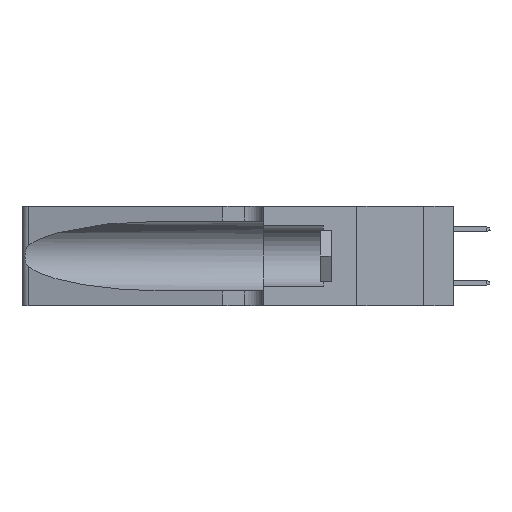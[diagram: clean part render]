
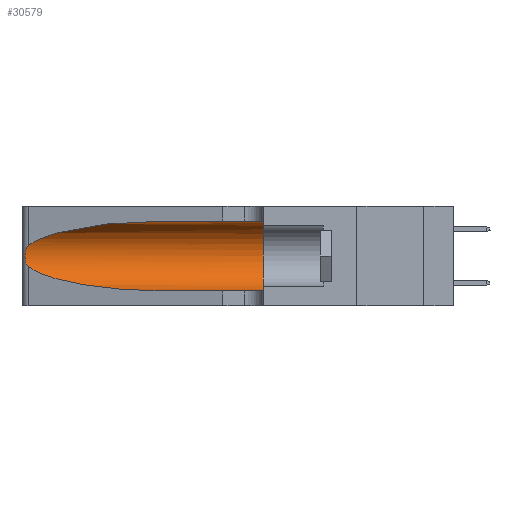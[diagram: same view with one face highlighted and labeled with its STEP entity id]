
A CAD part, left-side view. The second image highlights one B-rep face of the part: STEP entity #30579.
In plain terms, the highlighted cylindrical face has radius 3.308 mm (diameter 6.617 mm), a partial arc.
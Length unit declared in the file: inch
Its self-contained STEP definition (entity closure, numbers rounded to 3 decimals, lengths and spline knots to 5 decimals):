
#623 = CARTESIAN_POINT ( 'NONE',  ( 0.1305, 0.72297, 0.05475 ) ) ;
#977 = EDGE_CURVE ( 'NONE', #23095, #16569, #15857, .T. ) ;
#1763 = CARTESIAN_POINT ( 'NONE',  ( 0.25854, 1.2359, 0.20912 ) ) ;
#2706 = EDGE_CURVE ( 'NONE', #24410, #31157, #18891, .T. ) ;
#2961 = CARTESIAN_POINT ( 'NONE',  ( 0.2373, 1.15595, 0.28018 ) ) ;
#3534 = DIRECTION ( 'NONE',  ( 0., -1., 0. ) ) ;
#4025 = B_SPLINE_CURVE_WITH_KNOTS ( 'NONE', 3,
 ( #13076, #18760, #31035, #4410, #1763, #33311, #21783, #10245, #13274, #4963, #24833, #36332, #10434, #16480 ),
 .UNSPECIFIED., .F., .F.,
 ( 4, 2, 2, 2, 2, 2, 4 ),
 ( 0., 0.00027, 0.00053, 0.00107, 0.0016, 0.00187, 0.00214 ),
 .UNSPECIFIED. ) ;
#4410 = CARTESIAN_POINT ( 'NONE',  ( 0.25787, 1.23484, 0.2124 ) ) ;
#4963 = CARTESIAN_POINT ( 'NONE',  ( 0.25856, 1.23593, 0.16098 ) ) ;
#6735 = ORIENTED_EDGE ( 'NONE', *, *, #34462, .T. ) ;
#7719 = DIRECTION ( 'NONE',  ( 0., 1., 0. ) ) ;
#10245 = CARTESIAN_POINT ( 'NONE',  ( 0.26075, 1.23896, 0.178 ) ) ;
#10434 = CARTESIAN_POINT ( 'NONE',  ( 0.25555, 1.22993, 0.14849 ) ) ;
#10559 = ORIENTED_EDGE ( 'NONE', *, *, #21443, .T. ) ;
#11405 = ORIENTED_EDGE ( 'NONE', *, *, #977, .T. ) ;
#11571 = CARTESIAN_POINT ( 'NONE',  ( 0.18966, 0.96281, 0.05475 ) ) ;
#13076 = CARTESIAN_POINT ( 'NONE',  ( 0.25487, 1.22718, 0.22369 ) ) ;
#13154 = CARTESIAN_POINT ( 'NONE',  ( 0.1305, 0.72297, 0.05475 ) ) ;
#13274 = CARTESIAN_POINT ( 'NONE',  ( 0.26017, 1.23833, 0.17102 ) ) ;
#13378 = CARTESIAN_POINT ( 'NONE',  ( 0.1305, 0.35, 0.185 ) ) ;
#13765 = DIRECTION ( 'NONE',  ( 0., 0., -1. ) ) ;
#14661 = CARTESIAN_POINT ( 'NONE',  ( 0.18966, 0.96281, 0.31525 ) ) ;
#14711 = VERTEX_POINT ( 'NONE', #26350 ) ;
#14778 = CARTESIAN_POINT ( 'NONE',  ( 0.25487, 1.22718, 0.14631 ) ) ;
#15183 = EDGE_CURVE ( 'NONE', #23095, #24410, #29233, .T. ) ;
#15538 = ORIENTED_EDGE ( 'NONE', *, *, #26719, .T. ) ;
#15857 =( BOUNDED_CURVE ( )  B_SPLINE_CURVE ( 3, ( #35417, #14661, #2961, #29213 ),
 .UNSPECIFIED., .F., .T. ) 
 B_SPLINE_CURVE_WITH_KNOTS ( ( 4, 4 ),
 ( 1.5708, 2.84003 ),
 .UNSPECIFIED. ) 
 CURVE ( )  GEOMETRIC_REPRESENTATION_ITEM ( )  RATIONAL_B_SPLINE_CURVE ( ( 1., 0.87, 0.87, 1. ) ) 
 REPRESENTATION_ITEM ( '' )  );
#16031 = DIRECTION ( 'NONE',  ( 0., -1., 0. ) ) ;
#16468 = AXIS2_PLACEMENT_3D ( 'NONE', #13378, #7719, #24936 ) ;
#16480 = CARTESIAN_POINT ( 'NONE',  ( 0.25487, 1.22718, 0.14631 ) ) ;
#16569 = VERTEX_POINT ( 'NONE', #16725 ) ;
#16725 = CARTESIAN_POINT ( 'NONE',  ( 0.25487, 1.22718, 0.22369 ) ) ;
#16978 = DIRECTION ( 'NONE',  ( 0., -1., 0. ) ) ;
#17328 = VECTOR ( 'NONE', #16031, 39.37008 ) ;
#18760 = CARTESIAN_POINT ( 'NONE',  ( 0.25555, 1.22994, 0.2215 ) ) ;
#18891 = CIRCLE ( 'NONE', #16468, 0.13025 ) ;
#21308 = VECTOR ( 'NONE', #3534, 39.37008 ) ;
#21443 = EDGE_CURVE ( 'NONE', #21838, #31157, #30611, .T. ) ;
#21783 = CARTESIAN_POINT ( 'NONE',  ( 0.26075, 1.23896, 0.19203 ) ) ;
#21838 = VERTEX_POINT ( 'NONE', #13154 ) ;
#21991 = ORIENTED_EDGE ( 'NONE', *, *, #15183, .F. ) ;
#23095 = VERTEX_POINT ( 'NONE', #26203 ) ;
#24410 = VERTEX_POINT ( 'NONE', #27912 ) ;
#24833 = CARTESIAN_POINT ( 'NONE',  ( 0.25789, 1.23486, 0.15765 ) ) ;
#24936 = DIRECTION ( 'NONE',  ( 0., 0., 1. ) ) ;
#24941 = FACE_OUTER_BOUND ( 'NONE', #29448, .T. ) ;
#25057 =( BOUNDED_CURVE ( )  B_SPLINE_CURVE ( 3, ( #14778, #26507, #11571, #623 ),
 .UNSPECIFIED., .F., .T. ) 
 B_SPLINE_CURVE_WITH_KNOTS ( ( 4, 4 ),
 ( 3.44316, 4.71239 ),
 .UNSPECIFIED. ) 
 CURVE ( )  GEOMETRIC_REPRESENTATION_ITEM ( )  RATIONAL_B_SPLINE_CURVE ( ( 1., 0.87, 0.87, 1. ) ) 
 REPRESENTATION_ITEM ( '' )  );
#25085 = AXIS2_PLACEMENT_3D ( 'NONE', #27962, #16978, #13765 ) ;
#26203 = CARTESIAN_POINT ( 'NONE',  ( 0.1305, 0.72297, 0.31525 ) ) ;
#26350 = CARTESIAN_POINT ( 'NONE',  ( 0.25487, 1.22718, 0.14631 ) ) ;
#26437 = ORIENTED_EDGE ( 'NONE', *, *, #2706, .F. ) ;
#26507 = CARTESIAN_POINT ( 'NONE',  ( 0.2373, 1.15595, 0.08982 ) ) ;
#26719 = EDGE_CURVE ( 'NONE', #16569, #14711, #4025, .T. ) ;
#26933 = CARTESIAN_POINT ( 'NONE',  ( 0.1305, 0.35, 0.05475 ) ) ;
#27912 = CARTESIAN_POINT ( 'NONE',  ( 0.1305, 0.35, 0.31525 ) ) ;
#27962 = CARTESIAN_POINT ( 'NONE',  ( 0.1305, 1.61858, 0.185 ) ) ;
#29213 = CARTESIAN_POINT ( 'NONE',  ( 0.25487, 1.22718, 0.22369 ) ) ;
#29233 = LINE ( 'NONE', #29429, #21308 ) ;
#29429 = CARTESIAN_POINT ( 'NONE',  ( 0.1305, 1.61858, 0.31525 ) ) ;
#29448 = EDGE_LOOP ( 'NONE', ( #11405, #15538, #6735, #10559, #26437, #21991 ) ) ;
#30579 = ADVANCED_FACE ( 'NONE', ( #24941 ), #30788, .F. ) ;
#30611 = LINE ( 'NONE', #33614, #17328 ) ;
#30788 = CYLINDRICAL_SURFACE ( 'NONE', #25085, 0.13025 ) ;
#31035 = CARTESIAN_POINT ( 'NONE',  ( 0.25639, 1.23184, 0.21858 ) ) ;
#31157 = VERTEX_POINT ( 'NONE', #26933 ) ;
#33311 = CARTESIAN_POINT ( 'NONE',  ( 0.26018, 1.23835, 0.19895 ) ) ;
#33614 = CARTESIAN_POINT ( 'NONE',  ( 0.1305, 1.61858, 0.05475 ) ) ;
#34462 = EDGE_CURVE ( 'NONE', #14711, #21838, #25057, .T. ) ;
#35417 = CARTESIAN_POINT ( 'NONE',  ( 0.1305, 0.72297, 0.31525 ) ) ;
#36332 = CARTESIAN_POINT ( 'NONE',  ( 0.25639, 1.23186, 0.15144 ) ) ;
